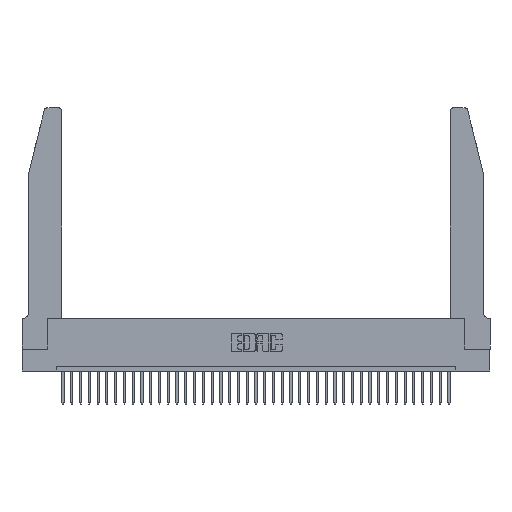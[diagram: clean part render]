
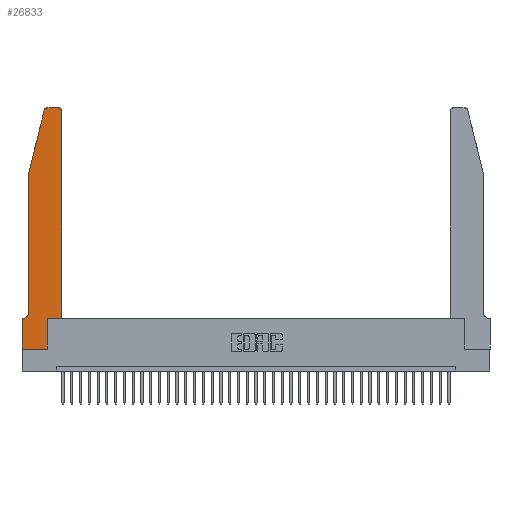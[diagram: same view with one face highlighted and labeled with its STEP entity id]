
A CAD part, top view. The second image highlights one B-rep face of the part: STEP entity #26833.
In plain terms, the highlighted planar face has unit normal (0, 0, 1).
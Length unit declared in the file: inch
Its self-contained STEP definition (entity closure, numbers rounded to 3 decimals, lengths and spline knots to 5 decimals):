
#103 = AXIS2_PLACEMENT_3D ( 'NONE', #10541, #7671, #22337 ) ;
#653 = VERTEX_POINT ( 'NONE', #17921 ) ;
#1197 = PLANE ( 'NONE',  #25871 ) ;
#1301 = CARTESIAN_POINT ( 'NONE',  ( 0.4505, 0.35, 0.37 ) ) ;
#1687 = DIRECTION ( 'NONE',  ( 0., 1., 0. ) ) ;
#1849 = VERTEX_POINT ( 'NONE', #27329 ) ;
#1955 = LINE ( 'NONE', #28407, #19068 ) ;
#3123 = DIRECTION ( 'NONE',  ( 0., -1., 0. ) ) ;
#3224 = EDGE_CURVE ( 'NONE', #4681, #33008, #26462, .T. ) ;
#3782 = EDGE_CURVE ( 'NONE', #34310, #26762, #21425, .T. ) ;
#3828 = VERTEX_POINT ( 'NONE', #37440 ) ;
#4681 = VERTEX_POINT ( 'NONE', #11248 ) ;
#4969 = ORIENTED_EDGE ( 'NONE', *, *, #35511, .T. ) ;
#5589 = ORIENTED_EDGE ( 'NONE', *, *, #27144, .T. ) ;
#5948 = EDGE_CURVE ( 'NONE', #7346, #9303, #16236, .T. ) ;
#6082 = DIRECTION ( 'NONE',  ( -1., 0., 0. ) ) ;
#6467 = VERTEX_POINT ( 'NONE', #29101 ) ;
#7005 = EDGE_CURVE ( 'NONE', #1849, #4681, #17520, .T. ) ;
#7209 = ORIENTED_EDGE ( 'NONE', *, *, #3782, .T. ) ;
#7346 = VERTEX_POINT ( 'NONE', #8787 ) ;
#7671 = DIRECTION ( 'NONE',  ( 0., 0., 1. ) ) ;
#8462 = VECTOR ( 'NONE', #8812, 39.37008 ) ;
#8484 = VECTOR ( 'NONE', #21217, 39.37008 ) ;
#8787 = CARTESIAN_POINT ( 'NONE',  ( 0.0055, 0.35, 0.37 ) ) ;
#8812 = DIRECTION ( 'NONE',  ( 0., 1., 0. ) ) ;
#8816 = ORIENTED_EDGE ( 'NONE', *, *, #7005, .T. ) ;
#9303 = VERTEX_POINT ( 'NONE', #36539 ) ;
#9333 = CARTESIAN_POINT ( 'NONE',  ( 0., 0., 0.37 ) ) ;
#9393 = ORIENTED_EDGE ( 'NONE', *, *, #30135, .T. ) ;
#10435 = VECTOR ( 'NONE', #31550, 39.37008 ) ;
#10517 = EDGE_CURVE ( 'NONE', #25885, #653, #37550, .T. ) ;
#10541 = CARTESIAN_POINT ( 'NONE',  ( 0.4205, 2.72, 0.37 ) ) ;
#11156 = EDGE_CURVE ( 'NONE', #3828, #22404, #1955, .T. ) ;
#11163 = EDGE_CURVE ( 'NONE', #653, #1849, #15349, .T. ) ;
#11248 = CARTESIAN_POINT ( 'NONE',  ( 0.4505, 0.35, 0.37 ) ) ;
#11465 = AXIS2_PLACEMENT_3D ( 'NONE', #14147, #25790, #31605 ) ;
#11628 = FACE_OUTER_BOUND ( 'NONE', #27531, .T. ) ;
#12486 = ORIENTED_EDGE ( 'NONE', *, *, #17190, .T. ) ;
#12873 = DIRECTION ( 'NONE',  ( -0.239, -0.971, 0. ) ) ;
#13008 = ORIENTED_EDGE ( 'NONE', *, *, #3224, .T. ) ;
#13582 = DIRECTION ( 'NONE',  ( 1., 0., 0. ) ) ;
#14095 = CARTESIAN_POINT ( 'NONE',  ( 0.4505, 0.35, 0.37 ) ) ;
#14147 = CARTESIAN_POINT ( 'NONE',  ( 0.284, 2.72, 0.37 ) ) ;
#15280 = AXIS2_PLACEMENT_3D ( 'NONE', #20359, #35238, #35486 ) ;
#15349 = LINE ( 'NONE', #16645, #23206 ) ;
#16236 = LINE ( 'NONE', #32556, #34275 ) ;
#16645 = CARTESIAN_POINT ( 'NONE',  ( 0.2865, 0.35, 0.37 ) ) ;
#17190 = EDGE_CURVE ( 'NONE', #33008, #3828, #30463, .T. ) ;
#17520 = LINE ( 'NONE', #1301, #23065 ) ;
#17921 = CARTESIAN_POINT ( 'NONE',  ( 0.2865, 0., 0.37 ) ) ;
#18414 = ORIENTED_EDGE ( 'NONE', *, *, #5948, .T. ) ;
#19068 = VECTOR ( 'NONE', #31257, 39.37008 ) ;
#19662 = ORIENTED_EDGE ( 'NONE', *, *, #11156, .T. ) ;
#19949 = ORIENTED_EDGE ( 'NONE', *, *, #11163, .T. ) ;
#20156 = CARTESIAN_POINT ( 'NONE',  ( 0.0755, 2., 0.37 ) ) ;
#20359 = CARTESIAN_POINT ( 'NONE',  ( 0.0055, 0.42, 0.37 ) ) ;
#20474 = CARTESIAN_POINT ( 'NONE',  ( 0., 0., 0.37 ) ) ;
#21217 = DIRECTION ( 'NONE',  ( 1., 0., 0. ) ) ;
#21425 = LINE ( 'NONE', #31673, #10435 ) ;
#21469 = CIRCLE ( 'NONE', #11465, 0.03 ) ;
#22337 = DIRECTION ( 'NONE',  ( 1., 0., 0. ) ) ;
#22404 = VERTEX_POINT ( 'NONE', #37589 ) ;
#22920 = CIRCLE ( 'NONE', #15280, 0.07 ) ;
#23065 = VECTOR ( 'NONE', #13582, 39.37008 ) ;
#23206 = VECTOR ( 'NONE', #1687, 39.37008 ) ;
#23705 = ORIENTED_EDGE ( 'NONE', *, *, #10517, .T. ) ;
#24439 = CARTESIAN_POINT ( 'NONE',  ( 0.0755, 0.42, 0.37 ) ) ;
#24496 = CARTESIAN_POINT ( 'NONE',  ( 0.0755, 2., 0.37 ) ) ;
#25093 = CARTESIAN_POINT ( 'NONE',  ( 0., 0.35, 0.37 ) ) ;
#25790 = DIRECTION ( 'NONE',  ( 0., 0., 1. ) ) ;
#25871 = AXIS2_PLACEMENT_3D ( 'NONE', #25093, #27536, #31030 ) ;
#25885 = VERTEX_POINT ( 'NONE', #26203 ) ;
#26203 = CARTESIAN_POINT ( 'NONE',  ( 0., 0., 0.37 ) ) ;
#26462 = LINE ( 'NONE', #14095, #8462 ) ;
#26762 = VERTEX_POINT ( 'NONE', #24439 ) ;
#26833 = ADVANCED_FACE ( 'NONE', ( #11628 ), #1197, .T. ) ;
#27144 = EDGE_CURVE ( 'NONE', #9303, #25885, #35610, .T. ) ;
#27329 = CARTESIAN_POINT ( 'NONE',  ( 0.2865, 0.35, 0.37 ) ) ;
#27531 = EDGE_LOOP ( 'NONE', ( #19662, #4969, #37209, #7209, #9393, #18414, #5589, #23705, #19949, #8816, #13008, #12486 ) ) ;
#27536 = DIRECTION ( 'NONE',  ( 0., 0., 1. ) ) ;
#27765 = EDGE_CURVE ( 'NONE', #6467, #34310, #31397, .T. ) ;
#28407 = CARTESIAN_POINT ( 'NONE',  ( 0.2605, 2.75, 0.37 ) ) ;
#29101 = CARTESIAN_POINT ( 'NONE',  ( 0.25487, 2.72718, 0.37 ) ) ;
#30049 = VECTOR ( 'NONE', #3123, 39.37008 ) ;
#30135 = EDGE_CURVE ( 'NONE', #26762, #7346, #22920, .T. ) ;
#30456 = VECTOR ( 'NONE', #12873, 39.37008 ) ;
#30463 = CIRCLE ( 'NONE', #103, 0.03 ) ;
#31030 = DIRECTION ( 'NONE',  ( 1., 0., 0. ) ) ;
#31243 = CARTESIAN_POINT ( 'NONE',  ( 0.4505, 2.72, 0.37 ) ) ;
#31257 = DIRECTION ( 'NONE',  ( -1., 0., 0. ) ) ;
#31397 = LINE ( 'NONE', #24496, #30456 ) ;
#31550 = DIRECTION ( 'NONE',  ( 0., -1., 0. ) ) ;
#31605 = DIRECTION ( 'NONE',  ( 1., 0., 0. ) ) ;
#31673 = CARTESIAN_POINT ( 'NONE',  ( 0.0755, 2., 0.37 ) ) ;
#32556 = CARTESIAN_POINT ( 'NONE',  ( 0.0755, 0.35, 0.37 ) ) ;
#33008 = VERTEX_POINT ( 'NONE', #31243 ) ;
#34275 = VECTOR ( 'NONE', #6082, 39.37008 ) ;
#34310 = VERTEX_POINT ( 'NONE', #20156 ) ;
#35238 = DIRECTION ( 'NONE',  ( 0., 0., -1. ) ) ;
#35486 = DIRECTION ( 'NONE',  ( -1., 0., 0. ) ) ;
#35511 = EDGE_CURVE ( 'NONE', #22404, #6467, #21469, .T. ) ;
#35610 = LINE ( 'NONE', #9333, #30049 ) ;
#36539 = CARTESIAN_POINT ( 'NONE',  ( 0., 0.35, 0.37 ) ) ;
#37209 = ORIENTED_EDGE ( 'NONE', *, *, #27765, .T. ) ;
#37440 = CARTESIAN_POINT ( 'NONE',  ( 0.4205, 2.75, 0.37 ) ) ;
#37550 = LINE ( 'NONE', #20474, #8484 ) ;
#37589 = CARTESIAN_POINT ( 'NONE',  ( 0.284, 2.75, 0.37 ) ) ;
